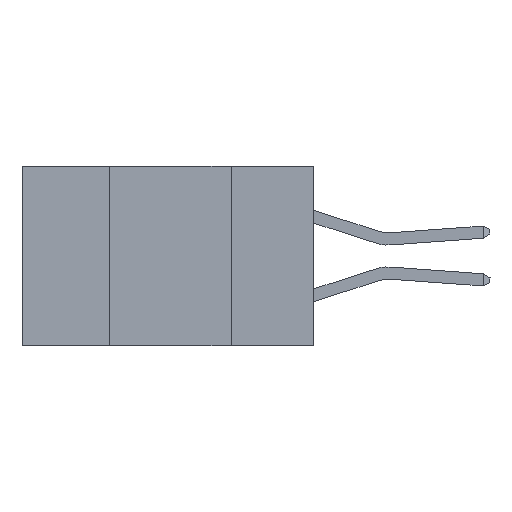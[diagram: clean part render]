
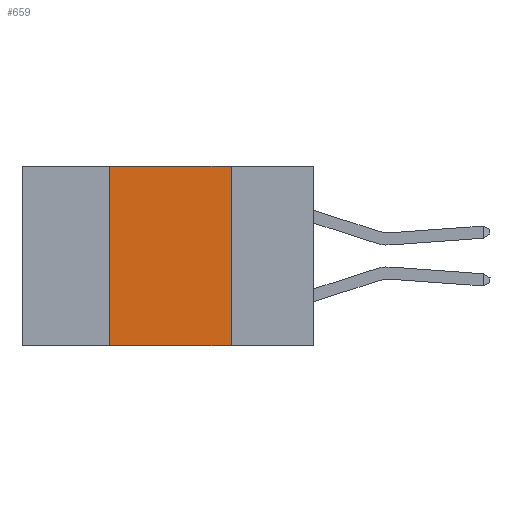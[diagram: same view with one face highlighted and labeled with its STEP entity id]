
A CAD part, left-side view. The second image highlights one B-rep face of the part: STEP entity #659.
In plain terms, the highlighted planar face has unit normal (-1, 0, 0).
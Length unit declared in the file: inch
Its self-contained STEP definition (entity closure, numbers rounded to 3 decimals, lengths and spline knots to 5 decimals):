
#203 = VECTOR ( 'NONE', #1852, 39.37008 ) ;
#583 = VECTOR ( 'NONE', #16508, 39.37008 ) ;
#659 = ADVANCED_FACE ( 'NONE', ( #21391 ), #5348, .F. ) ;
#1309 = VERTEX_POINT ( 'NONE', #19274 ) ;
#1852 = DIRECTION ( 'NONE',  ( 0., -1., 0. ) ) ;
#2095 = VERTEX_POINT ( 'NONE', #19047 ) ;
#2257 = EDGE_CURVE ( 'NONE', #7109, #1309, #13719, .T. ) ;
#5348 = PLANE ( 'NONE',  #12071 ) ;
#5676 = CARTESIAN_POINT ( 'NONE',  ( 0., 0.42, 0. ) ) ;
#5982 = CARTESIAN_POINT ( 'NONE',  ( 0., 0.6, 0. ) ) ;
#7109 = VERTEX_POINT ( 'NONE', #9890 ) ;
#8252 = DIRECTION ( 'NONE',  ( 1., 0., 0. ) ) ;
#8437 = DIRECTION ( 'NONE',  ( 0., 0., -1. ) ) ;
#8446 = VERTEX_POINT ( 'NONE', #10218 ) ;
#8497 = CARTESIAN_POINT ( 'NONE',  ( 0., 0.6, 0. ) ) ;
#9437 = LINE ( 'NONE', #5982, #583 ) ;
#9890 = CARTESIAN_POINT ( 'NONE',  ( 0., 0.42, -0.37 ) ) ;
#10218 = CARTESIAN_POINT ( 'NONE',  ( 0., 0.42, 0. ) ) ;
#11758 = EDGE_LOOP ( 'NONE', ( #14727, #20047, #18650, #16625 ) ) ;
#11962 = CARTESIAN_POINT ( 'NONE',  ( 0., 0.17, 0. ) ) ;
#12071 = AXIS2_PLACEMENT_3D ( 'NONE', #8497, #8252, #21506 ) ;
#12892 = VECTOR ( 'NONE', #17942, 39.37008 ) ;
#13719 = LINE ( 'NONE', #13760, #203 ) ;
#13760 = CARTESIAN_POINT ( 'NONE',  ( 0., 0.6, -0.37 ) ) ;
#14727 = ORIENTED_EDGE ( 'NONE', *, *, #19328, .F. ) ;
#16508 = DIRECTION ( 'NONE',  ( 0., -1., 0. ) ) ;
#16625 = ORIENTED_EDGE ( 'NONE', *, *, #2257, .T. ) ;
#17461 = LINE ( 'NONE', #5676, #12892 ) ;
#17942 = DIRECTION ( 'NONE',  ( 0., 0., 1. ) ) ;
#18328 = EDGE_CURVE ( 'NONE', #8446, #2095, #9437, .T. ) ;
#18650 = ORIENTED_EDGE ( 'NONE', *, *, #20902, .F. ) ;
#19047 = CARTESIAN_POINT ( 'NONE',  ( 0., 0.17, 0. ) ) ;
#19274 = CARTESIAN_POINT ( 'NONE',  ( 0., 0.17, -0.37 ) ) ;
#19328 = EDGE_CURVE ( 'NONE', #2095, #1309, #20005, .T. ) ;
#19474 = VECTOR ( 'NONE', #8437, 39.37008 ) ;
#20005 = LINE ( 'NONE', #11962, #19474 ) ;
#20047 = ORIENTED_EDGE ( 'NONE', *, *, #18328, .F. ) ;
#20902 = EDGE_CURVE ( 'NONE', #7109, #8446, #17461, .T. ) ;
#21391 = FACE_OUTER_BOUND ( 'NONE', #11758, .T. ) ;
#21506 = DIRECTION ( 'NONE',  ( 0., 0., -1. ) ) ;
